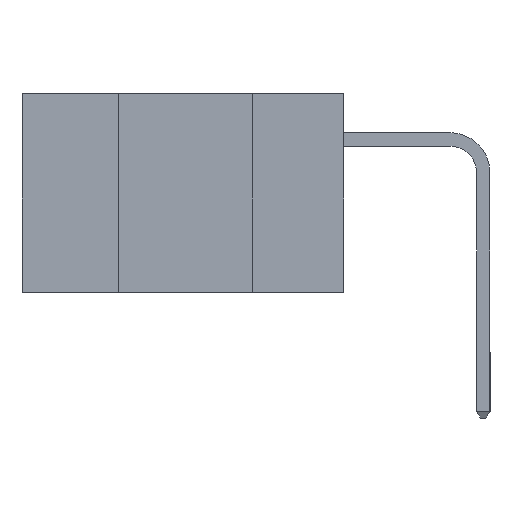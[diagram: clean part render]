
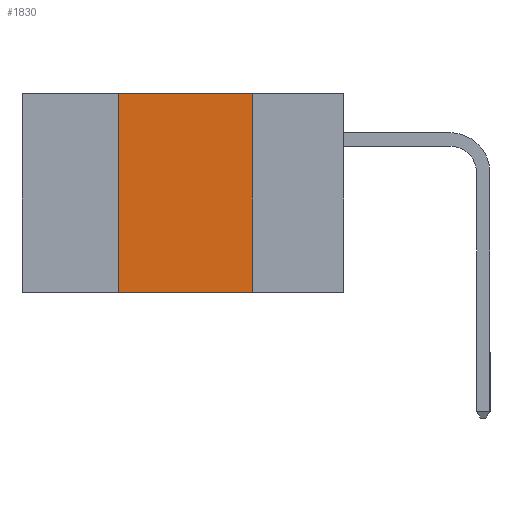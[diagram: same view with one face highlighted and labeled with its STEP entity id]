
A CAD part, left-side view. The second image highlights one B-rep face of the part: STEP entity #1830.
In plain terms, the highlighted planar face has unit normal (-1, 0, 0).
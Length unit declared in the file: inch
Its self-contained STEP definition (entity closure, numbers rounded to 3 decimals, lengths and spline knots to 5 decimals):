
#249 = DIRECTION ( 'NONE',  ( 0., 0., -1. ) ) ;
#475 = VECTOR ( 'NONE', #12299, 39.37008 ) ;
#692 = CARTESIAN_POINT ( 'NONE',  ( 0., 0.6, -0.37 ) ) ;
#827 = DIRECTION ( 'NONE',  ( 1., 0., 0. ) ) ;
#884 = CARTESIAN_POINT ( 'NONE',  ( 0., 0.42, -0.37 ) ) ;
#1332 = EDGE_LOOP ( 'NONE', ( #8868, #2012, #7618, #11833 ) ) ;
#1830 = ADVANCED_FACE ( 'NONE', ( #7475 ), #6351, .F. ) ;
#2012 = ORIENTED_EDGE ( 'NONE', *, *, #4373, .F. ) ;
#2565 = VERTEX_POINT ( 'NONE', #11391 ) ;
#2751 = LINE ( 'NONE', #884, #9270 ) ;
#3139 = VECTOR ( 'NONE', #7405, 39.37008 ) ;
#3244 = EDGE_CURVE ( 'NONE', #2565, #9206, #2751, .T. ) ;
#3361 = LINE ( 'NONE', #8858, #10761 ) ;
#4373 = EDGE_CURVE ( 'NONE', #9206, #10879, #9429, .T. ) ;
#4879 = DIRECTION ( 'NONE',  ( 0., 0., 1. ) ) ;
#5697 = CARTESIAN_POINT ( 'NONE',  ( 0., 0.42, 0. ) ) ;
#6007 = EDGE_CURVE ( 'NONE', #2565, #7661, #11182, .T. ) ;
#6351 = PLANE ( 'NONE',  #6495 ) ;
#6407 = CARTESIAN_POINT ( 'NONE',  ( 0., 0.6, 0. ) ) ;
#6495 = AXIS2_PLACEMENT_3D ( 'NONE', #6407, #827, #11193 ) ;
#7011 = CARTESIAN_POINT ( 'NONE',  ( 0., 0.17, 0. ) ) ;
#7405 = DIRECTION ( 'NONE',  ( 0., -1., 0. ) ) ;
#7475 = FACE_OUTER_BOUND ( 'NONE', #1332, .T. ) ;
#7618 = ORIENTED_EDGE ( 'NONE', *, *, #3244, .F. ) ;
#7661 = VERTEX_POINT ( 'NONE', #7675 ) ;
#7675 = CARTESIAN_POINT ( 'NONE',  ( 0., 0.17, -0.37 ) ) ;
#8858 = CARTESIAN_POINT ( 'NONE',  ( 0., 0.17, -0.37 ) ) ;
#8868 = ORIENTED_EDGE ( 'NONE', *, *, #10528, .F. ) ;
#9206 = VERTEX_POINT ( 'NONE', #5697 ) ;
#9270 = VECTOR ( 'NONE', #4879, 39.37008 ) ;
#9429 = LINE ( 'NONE', #11377, #3139 ) ;
#10528 = EDGE_CURVE ( 'NONE', #10879, #7661, #3361, .T. ) ;
#10761 = VECTOR ( 'NONE', #249, 39.37008 ) ;
#10879 = VERTEX_POINT ( 'NONE', #7011 ) ;
#11182 = LINE ( 'NONE', #692, #475 ) ;
#11193 = DIRECTION ( 'NONE',  ( 0., 0., -1. ) ) ;
#11377 = CARTESIAN_POINT ( 'NONE',  ( 0., 0.6, 0. ) ) ;
#11391 = CARTESIAN_POINT ( 'NONE',  ( 0., 0.42, -0.37 ) ) ;
#11833 = ORIENTED_EDGE ( 'NONE', *, *, #6007, .T. ) ;
#12299 = DIRECTION ( 'NONE',  ( 0., -1., 0. ) ) ;
